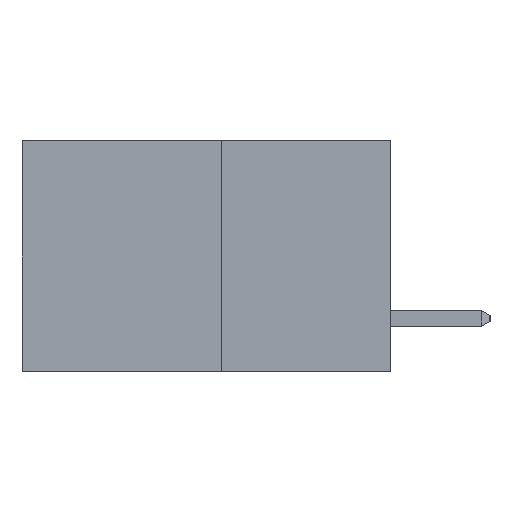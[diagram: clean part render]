
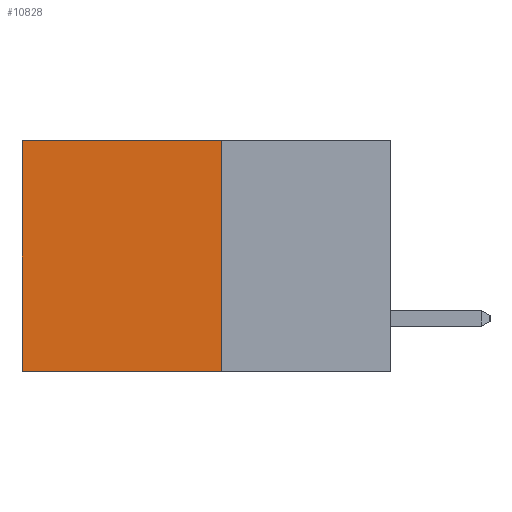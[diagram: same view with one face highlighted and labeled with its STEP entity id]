
A CAD part, left-side view. The second image highlights one B-rep face of the part: STEP entity #10828.
In plain terms, the highlighted planar face has unit normal (-1, 0, 0).
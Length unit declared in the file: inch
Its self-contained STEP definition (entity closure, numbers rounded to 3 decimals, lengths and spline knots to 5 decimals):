
#792 = DIRECTION ( 'NONE',  ( 0., 0., -1. ) ) ;
#813 = VERTEX_POINT ( 'NONE', #20190 ) ;
#822 = ORIENTED_EDGE ( 'NONE', *, *, #8345, .F. ) ;
#1956 = VECTOR ( 'NONE', #4733, 39.37008 ) ;
#2354 = DIRECTION ( 'NONE',  ( 0., 0., -1. ) ) ;
#3221 = ORIENTED_EDGE ( 'NONE', *, *, #11348, .T. ) ;
#3336 = CARTESIAN_POINT ( 'NONE',  ( 0.277, 0.27, -0.37 ) ) ;
#3528 = VECTOR ( 'NONE', #5221, 39.37008 ) ;
#4005 = CARTESIAN_POINT ( 'NONE',  ( 0.277, 0.27, 0. ) ) ;
#4733 = DIRECTION ( 'NONE',  ( 0., 0., -1. ) ) ;
#5221 = DIRECTION ( 'NONE',  ( 0., 1., 0. ) ) ;
#6387 = PLANE ( 'NONE',  #14639 ) ;
#7659 = VERTEX_POINT ( 'NONE', #8921 ) ;
#8345 = EDGE_CURVE ( 'NONE', #813, #22464, #18500, .T. ) ;
#8921 = CARTESIAN_POINT ( 'NONE',  ( 0.277, 0.59, 0. ) ) ;
#9848 = LINE ( 'NONE', #4005, #13725 ) ;
#9941 = EDGE_CURVE ( 'NONE', #7659, #22464, #12311, .T. ) ;
#10828 = ADVANCED_FACE ( 'NONE', ( #16087 ), #6387, .F. ) ;
#11256 = CARTESIAN_POINT ( 'NONE',  ( 0.277, 0.59, -0.37 ) ) ;
#11348 = EDGE_CURVE ( 'NONE', #21821, #7659, #9848, .T. ) ;
#12100 = DIRECTION ( 'NONE',  ( 1., 0., 0. ) ) ;
#12311 = LINE ( 'NONE', #19241, #16706 ) ;
#13725 = VECTOR ( 'NONE', #22777, 39.37008 ) ;
#14116 = ORIENTED_EDGE ( 'NONE', *, *, #19581, .F. ) ;
#14639 = AXIS2_PLACEMENT_3D ( 'NONE', #23291, #12100, #792 ) ;
#16087 = FACE_OUTER_BOUND ( 'NONE', #23490, .T. ) ;
#16706 = VECTOR ( 'NONE', #2354, 39.37008 ) ;
#17787 = CARTESIAN_POINT ( 'NONE',  ( 0.277, 0.27, -0.37 ) ) ;
#18500 = LINE ( 'NONE', #3336, #3528 ) ;
#19241 = CARTESIAN_POINT ( 'NONE',  ( 0.277, 0.59, -0.37 ) ) ;
#19581 = EDGE_CURVE ( 'NONE', #21821, #813, #21931, .T. ) ;
#20190 = CARTESIAN_POINT ( 'NONE',  ( 0.277, 0.27, -0.37 ) ) ;
#20823 = CARTESIAN_POINT ( 'NONE',  ( 0.277, 0.27, 0. ) ) ;
#21821 = VERTEX_POINT ( 'NONE', #20823 ) ;
#21931 = LINE ( 'NONE', #17787, #1956 ) ;
#22464 = VERTEX_POINT ( 'NONE', #11256 ) ;
#22777 = DIRECTION ( 'NONE',  ( 0., 1., 0. ) ) ;
#23291 = CARTESIAN_POINT ( 'NONE',  ( 0.277, 0.27, -0.37 ) ) ;
#23345 = ORIENTED_EDGE ( 'NONE', *, *, #9941, .T. ) ;
#23490 = EDGE_LOOP ( 'NONE', ( #23345, #822, #14116, #3221 ) ) ;
